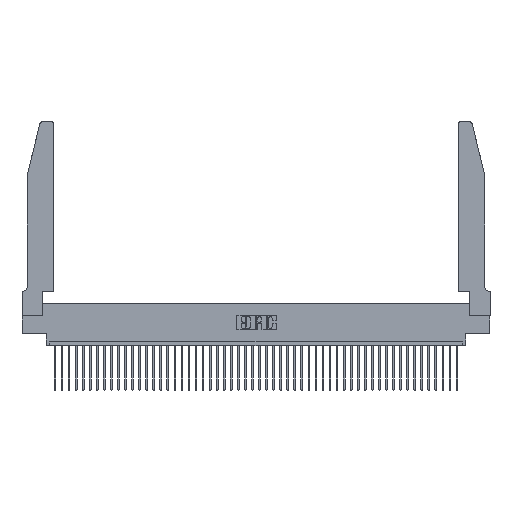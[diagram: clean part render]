
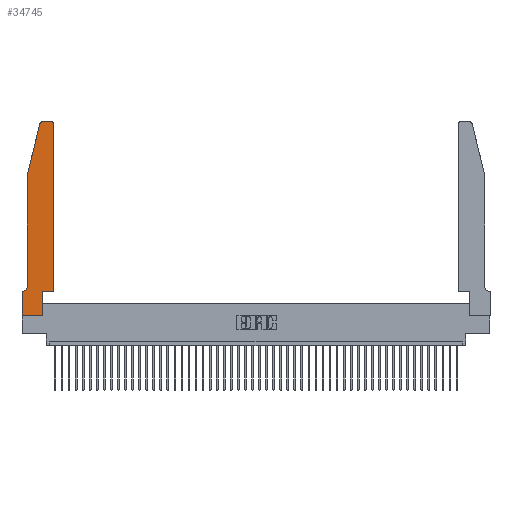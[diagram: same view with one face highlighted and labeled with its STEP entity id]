
A CAD part, top view. The second image highlights one B-rep face of the part: STEP entity #34745.
In plain terms, the highlighted planar face has unit normal (0, 0, 1).
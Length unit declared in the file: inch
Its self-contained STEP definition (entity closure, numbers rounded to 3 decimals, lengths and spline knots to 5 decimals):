
#438 = CARTESIAN_POINT ( 'NONE',  ( 0.0055, 0.42, 0.37 ) ) ;
#440 = VERTEX_POINT ( 'NONE', #17876 ) ;
#1009 = CARTESIAN_POINT ( 'NONE',  ( 0., 0.35, 0.37 ) ) ;
#1030 = VERTEX_POINT ( 'NONE', #17021 ) ;
#1452 = CARTESIAN_POINT ( 'NONE',  ( 0.0055, 0.35, 0.37 ) ) ;
#2603 = ORIENTED_EDGE ( 'NONE', *, *, #14239, .T. ) ;
#3032 = ORIENTED_EDGE ( 'NONE', *, *, #37084, .T. ) ;
#3192 = EDGE_CURVE ( 'NONE', #15993, #36032, #41313, .T. ) ;
#3917 = EDGE_LOOP ( 'NONE', ( #44996, #25421, #3032, #40512, #15349, #2603, #17271, #12594, #40435, #36946, #3952, #14620 ) ) ;
#3952 = ORIENTED_EDGE ( 'NONE', *, *, #25418, .T. ) ;
#4081 = EDGE_CURVE ( 'NONE', #42849, #36885, #8629, .T. ) ;
#4087 = DIRECTION ( 'NONE',  ( -1., 0., 0. ) ) ;
#4482 = DIRECTION ( 'NONE',  ( 0., 0., 1. ) ) ;
#4581 = AXIS2_PLACEMENT_3D ( 'NONE', #41774, #31440, #20452 ) ;
#4766 = EDGE_CURVE ( 'NONE', #18306, #26096, #33886, .T. ) ;
#4794 = LINE ( 'NONE', #11411, #44642 ) ;
#6952 = VECTOR ( 'NONE', #37085, 39.37008 ) ;
#7285 = FACE_OUTER_BOUND ( 'NONE', #3917, .T. ) ;
#7562 = CARTESIAN_POINT ( 'NONE',  ( 0.4505, 0.35, 0.37 ) ) ;
#7686 = DIRECTION ( 'NONE',  ( 0., 0., -1. ) ) ;
#8522 = EDGE_CURVE ( 'NONE', #440, #42849, #41020, .T. ) ;
#8629 = LINE ( 'NONE', #45023, #36201 ) ;
#8940 = CARTESIAN_POINT ( 'NONE',  ( 0.284, 2.75, 0.37 ) ) ;
#9356 = VECTOR ( 'NONE', #4087, 39.37008 ) ;
#10119 = LINE ( 'NONE', #19204, #40344 ) ;
#10783 = AXIS2_PLACEMENT_3D ( 'NONE', #1009, #4482, #15293 ) ;
#10837 = AXIS2_PLACEMENT_3D ( 'NONE', #438, #7686, #44504 ) ;
#11411 = CARTESIAN_POINT ( 'NONE',  ( 0.0755, 2., 0.37 ) ) ;
#11543 = EDGE_CURVE ( 'NONE', #1030, #15993, #24538, .T. ) ;
#12594 = ORIENTED_EDGE ( 'NONE', *, *, #8522, .T. ) ;
#13058 = VECTOR ( 'NONE', #44558, 39.37008 ) ;
#14239 = EDGE_CURVE ( 'NONE', #20291, #38337, #10119, .T. ) ;
#14620 = ORIENTED_EDGE ( 'NONE', *, *, #38447, .T. ) ;
#15293 = DIRECTION ( 'NONE',  ( 1., 0., 0. ) ) ;
#15349 = ORIENTED_EDGE ( 'NONE', *, *, #38170, .T. ) ;
#15993 = VERTEX_POINT ( 'NONE', #8940 ) ;
#16375 = CARTESIAN_POINT ( 'NONE',  ( 0.0755, 0.42, 0.37 ) ) ;
#16569 = CARTESIAN_POINT ( 'NONE',  ( 0., 0., 0.37 ) ) ;
#17021 = CARTESIAN_POINT ( 'NONE',  ( 0.4205, 2.75, 0.37 ) ) ;
#17271 = ORIENTED_EDGE ( 'NONE', *, *, #25568, .T. ) ;
#17876 = CARTESIAN_POINT ( 'NONE',  ( 0., 0., 0.37 ) ) ;
#18306 = VERTEX_POINT ( 'NONE', #23604 ) ;
#18610 = EDGE_CURVE ( 'NONE', #36885, #26460, #36575, .T. ) ;
#19204 = CARTESIAN_POINT ( 'NONE',  ( 0.0755, 0.35, 0.37 ) ) ;
#19304 = CIRCLE ( 'NONE', #10837, 0.07 ) ;
#19356 = CARTESIAN_POINT ( 'NONE',  ( 0.4505, 0.35, 0.37 ) ) ;
#19443 = CARTESIAN_POINT ( 'NONE',  ( 0.4505, 0.35, 0.37 ) ) ;
#19965 = CARTESIAN_POINT ( 'NONE',  ( 0., 0., 0.37 ) ) ;
#20291 = VERTEX_POINT ( 'NONE', #1452 ) ;
#20452 = DIRECTION ( 'NONE',  ( 1., 0., 0. ) ) ;
#21210 = LINE ( 'NONE', #19965, #34716 ) ;
#23604 = CARTESIAN_POINT ( 'NONE',  ( 0.0755, 2., 0.37 ) ) ;
#23731 = DIRECTION ( 'NONE',  ( 0., -1., 0. ) ) ;
#24184 = CARTESIAN_POINT ( 'NONE',  ( 0.4505, 2.72, 0.37 ) ) ;
#24538 = LINE ( 'NONE', #25587, #9356 ) ;
#25418 = EDGE_CURVE ( 'NONE', #26460, #37340, #46420, .T. ) ;
#25421 = ORIENTED_EDGE ( 'NONE', *, *, #3192, .T. ) ;
#25568 = EDGE_CURVE ( 'NONE', #38337, #440, #21210, .T. ) ;
#25587 = CARTESIAN_POINT ( 'NONE',  ( 0.2605, 2.75, 0.37 ) ) ;
#26096 = VERTEX_POINT ( 'NONE', #16375 ) ;
#26126 = DIRECTION ( 'NONE',  ( 1., 0., 0. ) ) ;
#26460 = VERTEX_POINT ( 'NONE', #19443 ) ;
#27244 = CARTESIAN_POINT ( 'NONE',  ( 0.25487, 2.72718, 0.37 ) ) ;
#27692 = CARTESIAN_POINT ( 'NONE',  ( 0.2865, 0.35, 0.37 ) ) ;
#27775 = CARTESIAN_POINT ( 'NONE',  ( 0.2865, 0., 0.37 ) ) ;
#30161 = CARTESIAN_POINT ( 'NONE',  ( 0.4205, 2.72, 0.37 ) ) ;
#30329 = DIRECTION ( 'NONE',  ( 1., 0., 0. ) ) ;
#30754 = VECTOR ( 'NONE', #44386, 39.37008 ) ;
#31440 = DIRECTION ( 'NONE',  ( 0., 0., 1. ) ) ;
#33175 = VECTOR ( 'NONE', #26126, 39.37008 ) ;
#33787 = DIRECTION ( 'NONE',  ( 0., 0., 1. ) ) ;
#33886 = LINE ( 'NONE', #44953, #6952 ) ;
#34716 = VECTOR ( 'NONE', #23731, 39.37008 ) ;
#34745 = ADVANCED_FACE ( 'NONE', ( #7285 ), #36682, .T. ) ;
#35641 = CIRCLE ( 'NONE', #46344, 0.03 ) ;
#36032 = VERTEX_POINT ( 'NONE', #27244 ) ;
#36201 = VECTOR ( 'NONE', #44696, 39.37008 ) ;
#36575 = LINE ( 'NONE', #19356, #13058 ) ;
#36682 = PLANE ( 'NONE',  #10783 ) ;
#36885 = VERTEX_POINT ( 'NONE', #27692 ) ;
#36946 = ORIENTED_EDGE ( 'NONE', *, *, #18610, .T. ) ;
#37084 = EDGE_CURVE ( 'NONE', #36032, #18306, #4794, .T. ) ;
#37085 = DIRECTION ( 'NONE',  ( 0., -1., 0. ) ) ;
#37340 = VERTEX_POINT ( 'NONE', #24184 ) ;
#38170 = EDGE_CURVE ( 'NONE', #26096, #20291, #19304, .T. ) ;
#38337 = VERTEX_POINT ( 'NONE', #39324 ) ;
#38447 = EDGE_CURVE ( 'NONE', #37340, #1030, #35641, .T. ) ;
#39324 = CARTESIAN_POINT ( 'NONE',  ( 0., 0.35, 0.37 ) ) ;
#40344 = VECTOR ( 'NONE', #44888, 39.37008 ) ;
#40435 = ORIENTED_EDGE ( 'NONE', *, *, #4081, .T. ) ;
#40512 = ORIENTED_EDGE ( 'NONE', *, *, #4766, .T. ) ;
#41020 = LINE ( 'NONE', #16569, #33175 ) ;
#41313 = CIRCLE ( 'NONE', #4581, 0.03 ) ;
#41774 = CARTESIAN_POINT ( 'NONE',  ( 0.284, 2.72, 0.37 ) ) ;
#42849 = VERTEX_POINT ( 'NONE', #27775 ) ;
#44386 = DIRECTION ( 'NONE',  ( 0., 1., 0. ) ) ;
#44504 = DIRECTION ( 'NONE',  ( -1., 0., 0. ) ) ;
#44558 = DIRECTION ( 'NONE',  ( 1., 0., 0. ) ) ;
#44642 = VECTOR ( 'NONE', #45592, 39.37008 ) ;
#44696 = DIRECTION ( 'NONE',  ( 0., 1., 0. ) ) ;
#44888 = DIRECTION ( 'NONE',  ( -1., 0., 0. ) ) ;
#44953 = CARTESIAN_POINT ( 'NONE',  ( 0.0755, 2., 0.37 ) ) ;
#44996 = ORIENTED_EDGE ( 'NONE', *, *, #11543, .T. ) ;
#45023 = CARTESIAN_POINT ( 'NONE',  ( 0.2865, 0.35, 0.37 ) ) ;
#45592 = DIRECTION ( 'NONE',  ( -0.239, -0.971, 0. ) ) ;
#46344 = AXIS2_PLACEMENT_3D ( 'NONE', #30161, #33787, #30329 ) ;
#46420 = LINE ( 'NONE', #7562, #30754 ) ;
